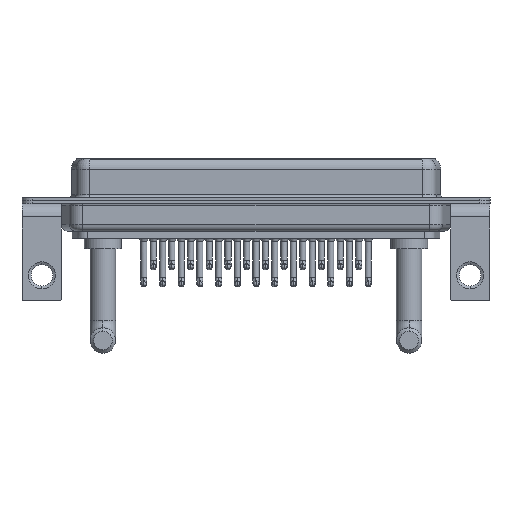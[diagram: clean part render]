
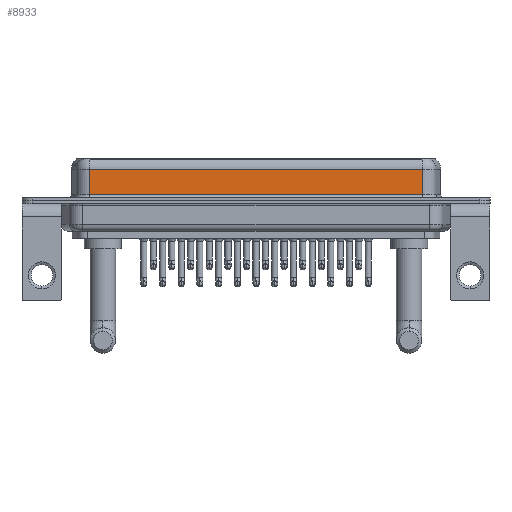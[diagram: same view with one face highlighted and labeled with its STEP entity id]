
A CAD part, front view. The second image highlights one B-rep face of the part: STEP entity #8933.
In plain terms, the highlighted planar face has unit normal (0, -1, 0).
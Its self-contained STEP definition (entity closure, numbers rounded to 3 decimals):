
#463 = VERTEX_POINT ( 'NONE', #14960 ) ;
#970 = VECTOR ( 'NONE', #11287, 1000. ) ;
#1855 = VECTOR ( 'NONE', #8988, 1000. ) ;
#1941 = LINE ( 'NONE', #5799, #22445 ) ;
#2014 = ORIENTED_EDGE ( 'NONE', *, *, #21293, .T. ) ;
#2956 = EDGE_CURVE ( 'NONE', #21858, #463, #1941, .T. ) ;
#3542 = CARTESIAN_POINT ( 'NONE',  ( 7.038, -3.95, 0.9 ) ) ;
#3774 = PLANE ( 'NONE',  #5293 ) ;
#4615 = DIRECTION ( 'NONE',  ( 0., 0., -1. ) ) ;
#5293 = AXIS2_PLACEMENT_3D ( 'NONE', #9881, #19564, #23589 ) ;
#5546 = EDGE_CURVE ( 'NONE', #20462, #6531, #11160, .T. ) ;
#5799 = CARTESIAN_POINT ( 'NONE',  ( 56.462, -3.95, 4.65 ) ) ;
#6302 = LINE ( 'NONE', #20040, #25032 ) ;
#6531 = VERTEX_POINT ( 'NONE', #15735 ) ;
#6879 = ORIENTED_EDGE ( 'NONE', *, *, #19068, .F. ) ;
#8933 = ADVANCED_FACE ( 'NONE', ( #15553 ), #3774, .F. ) ;
#8988 = DIRECTION ( 'NONE',  ( 0., 0., -1. ) ) ;
#9476 = CARTESIAN_POINT ( 'NONE',  ( 56.462, -3.95, 0.9 ) ) ;
#9854 = DIRECTION ( 'NONE',  ( -1., 0., 0. ) ) ;
#9881 = CARTESIAN_POINT ( 'NONE',  ( 56.462, -3.95, 6.4 ) ) ;
#11160 = LINE ( 'NONE', #9476, #970 ) ;
#11287 = DIRECTION ( 'NONE',  ( 1., 0., 0. ) ) ;
#14960 = CARTESIAN_POINT ( 'NONE',  ( 7.038, -3.95, 4.65 ) ) ;
#15553 = FACE_OUTER_BOUND ( 'NONE', #21516, .T. ) ;
#15735 = CARTESIAN_POINT ( 'NONE',  ( 56.462, -3.95, 0.9 ) ) ;
#19068 = EDGE_CURVE ( 'NONE', #21858, #6531, #20890, .T. ) ;
#19492 = ORIENTED_EDGE ( 'NONE', *, *, #2956, .T. ) ;
#19564 = DIRECTION ( 'NONE',  ( 0., 1., 0. ) ) ;
#20040 = CARTESIAN_POINT ( 'NONE',  ( 7.038, -3.95, 6.4 ) ) ;
#20462 = VERTEX_POINT ( 'NONE', #3542 ) ;
#20890 = LINE ( 'NONE', #22579, #1855 ) ;
#21293 = EDGE_CURVE ( 'NONE', #463, #20462, #6302, .T. ) ;
#21516 = EDGE_LOOP ( 'NONE', ( #6879, #19492, #2014, #22287 ) ) ;
#21858 = VERTEX_POINT ( 'NONE', #21949 ) ;
#21949 = CARTESIAN_POINT ( 'NONE',  ( 56.462, -3.95, 4.65 ) ) ;
#22287 = ORIENTED_EDGE ( 'NONE', *, *, #5546, .T. ) ;
#22445 = VECTOR ( 'NONE', #9854, 1000. ) ;
#22579 = CARTESIAN_POINT ( 'NONE',  ( 56.462, -3.95, 6.4 ) ) ;
#23589 = DIRECTION ( 'NONE',  ( 0., 0., 1. ) ) ;
#25032 = VECTOR ( 'NONE', #4615, 1000. ) ;
